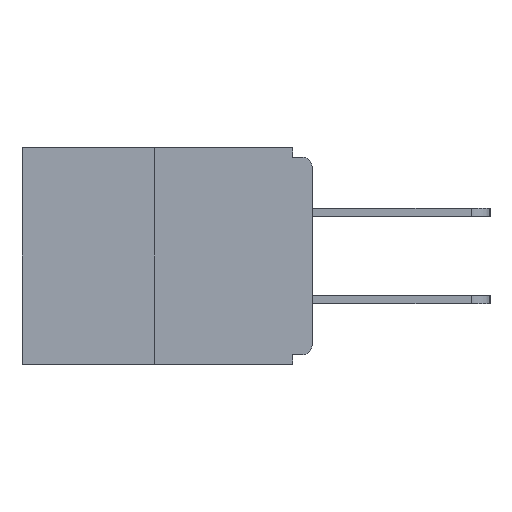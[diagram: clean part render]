
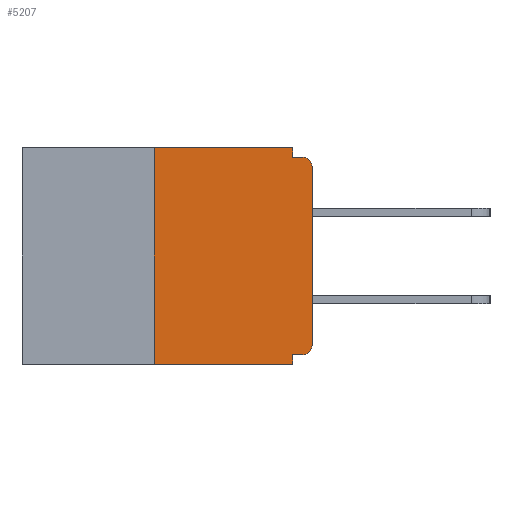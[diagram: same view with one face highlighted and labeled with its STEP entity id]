
A CAD part, left-side view. The second image highlights one B-rep face of the part: STEP entity #5207.
In plain terms, the highlighted planar face has unit normal (-1, 0, 0).
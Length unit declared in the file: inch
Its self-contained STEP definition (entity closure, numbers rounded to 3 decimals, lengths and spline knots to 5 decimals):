
#36 = ORIENTED_EDGE ( 'NONE', *, *, #3041, .F. ) ;
#191 = CARTESIAN_POINT ( 'NONE',  ( 0., 0.031, -0.328 ) ) ;
#299 = VECTOR ( 'NONE', #6464, 39.37008 ) ;
#502 = ORIENTED_EDGE ( 'NONE', *, *, #2843, .F. ) ;
#739 = EDGE_CURVE ( 'NONE', #14884, #6407, #12703, .T. ) ;
#771 = LINE ( 'NONE', #4756, #9662 ) ;
#773 = ORIENTED_EDGE ( 'NONE', *, *, #2170, .T. ) ;
#881 = LINE ( 'NONE', #10303, #8761 ) ;
#900 = LINE ( 'NONE', #12059, #10570 ) ;
#1342 = DIRECTION ( 'NONE',  ( 0., -1., 0. ) ) ;
#1424 = VERTEX_POINT ( 'NONE', #4488 ) ;
#1506 = VERTEX_POINT ( 'NONE', #13673 ) ;
#1543 = VERTEX_POINT ( 'NONE', #11147 ) ;
#1838 = ORIENTED_EDGE ( 'NONE', *, *, #739, .F. ) ;
#2103 = LINE ( 'NONE', #9027, #299 ) ;
#2170 = EDGE_CURVE ( 'NONE', #1424, #14766, #14477, .T. ) ;
#2428 = CARTESIAN_POINT ( 'NONE',  ( 0., 0.46, 0. ) ) ;
#2593 = VERTEX_POINT ( 'NONE', #6147 ) ;
#2674 = DIRECTION ( 'NONE',  ( 0., 0., -1. ) ) ;
#2838 = DIRECTION ( 'NONE',  ( 1., 0., 0. ) ) ;
#2843 = EDGE_CURVE ( 'NONE', #3686, #11981, #771, .T. ) ;
#3041 = EDGE_CURVE ( 'NONE', #1506, #1543, #13881, .T. ) ;
#3211 = CIRCLE ( 'NONE', #10064, 0.015 ) ;
#3686 = VERTEX_POINT ( 'NONE', #5465 ) ;
#3852 = DIRECTION ( 'NONE',  ( 0., 0., -1. ) ) ;
#4076 = AXIS2_PLACEMENT_3D ( 'NONE', #13822, #7461, #6131 ) ;
#4168 = DIRECTION ( 'NONE',  ( 0., 0., 1. ) ) ;
#4237 = EDGE_CURVE ( 'NONE', #14766, #2593, #5816, .T. ) ;
#4433 = ORIENTED_EDGE ( 'NONE', *, *, #15811, .T. ) ;
#4488 = CARTESIAN_POINT ( 'NONE',  ( 0., 0.015, -0.328 ) ) ;
#4657 = CARTESIAN_POINT ( 'NONE',  ( 0., 0.031, -0.343 ) ) ;
#4726 = EDGE_LOOP ( 'NONE', ( #36, #8362, #4433, #1838, #10491, #773, #16301, #13894, #502, #7622 ) ) ;
#4756 = CARTESIAN_POINT ( 'NONE',  ( 0., 0., -0.015 ) ) ;
#5207 = ADVANCED_FACE ( 'NONE', ( #11410 ), #7359, .F. ) ;
#5428 = DIRECTION ( 'NONE',  ( 0., 0., 1. ) ) ;
#5465 = CARTESIAN_POINT ( 'NONE',  ( 0., 0.031, -0.015 ) ) ;
#5483 = CARTESIAN_POINT ( 'NONE',  ( 0., 0., 0. ) ) ;
#5816 = LINE ( 'NONE', #5483, #12445 ) ;
#5883 = VECTOR ( 'NONE', #15792, 39.37008 ) ;
#6131 = DIRECTION ( 'NONE',  ( 0., 0., -1. ) ) ;
#6147 = CARTESIAN_POINT ( 'NONE',  ( 0., 0., -0.03 ) ) ;
#6407 = VERTEX_POINT ( 'NONE', #4657 ) ;
#6464 = DIRECTION ( 'NONE',  ( 0., 1., 0. ) ) ;
#6584 = CARTESIAN_POINT ( 'NONE',  ( 0., 0.015, -0.03 ) ) ;
#7234 = DIRECTION ( 'NONE',  ( 0., -1., 0. ) ) ;
#7359 = PLANE ( 'NONE',  #8649 ) ;
#7461 = DIRECTION ( 'NONE',  ( -1., 0., 0. ) ) ;
#7622 = ORIENTED_EDGE ( 'NONE', *, *, #11859, .F. ) ;
#8265 = VERTEX_POINT ( 'NONE', #16088 ) ;
#8362 = ORIENTED_EDGE ( 'NONE', *, *, #15459, .F. ) ;
#8649 = AXIS2_PLACEMENT_3D ( 'NONE', #10395, #2838, #2674 ) ;
#8681 = LINE ( 'NONE', #12797, #10885 ) ;
#8761 = VECTOR ( 'NONE', #1342, 39.37008 ) ;
#9027 = CARTESIAN_POINT ( 'NONE',  ( 0., 0., -0.328 ) ) ;
#9662 = VECTOR ( 'NONE', #7234, 39.37008 ) ;
#10064 = AXIS2_PLACEMENT_3D ( 'NONE', #6584, #12910, #15577 ) ;
#10303 = CARTESIAN_POINT ( 'NONE',  ( 0., 0.46, -0.343 ) ) ;
#10395 = CARTESIAN_POINT ( 'NONE',  ( 0., 0.46, 0. ) ) ;
#10491 = ORIENTED_EDGE ( 'NONE', *, *, #14849, .F. ) ;
#10570 = VECTOR ( 'NONE', #4168, 39.37008 ) ;
#10600 = CARTESIAN_POINT ( 'NONE',  ( 0., 0.031, -0.343 ) ) ;
#10885 = VECTOR ( 'NONE', #3852, 39.37008 ) ;
#11147 = CARTESIAN_POINT ( 'NONE',  ( 0., 0.031, 0. ) ) ;
#11410 = FACE_OUTER_BOUND ( 'NONE', #4726, .T. ) ;
#11806 = EDGE_CURVE ( 'NONE', #2593, #11981, #3211, .T. ) ;
#11859 = EDGE_CURVE ( 'NONE', #1543, #3686, #8681, .T. ) ;
#11981 = VERTEX_POINT ( 'NONE', #13239 ) ;
#12059 = CARTESIAN_POINT ( 'NONE',  ( 0., 0.25, 0. ) ) ;
#12445 = VECTOR ( 'NONE', #5428, 39.37008 ) ;
#12703 = LINE ( 'NONE', #10600, #5883 ) ;
#12797 = CARTESIAN_POINT ( 'NONE',  ( 0., 0.031, 0. ) ) ;
#12910 = DIRECTION ( 'NONE',  ( -1., 0., 0. ) ) ;
#13239 = CARTESIAN_POINT ( 'NONE',  ( 0., 0.015, -0.015 ) ) ;
#13673 = CARTESIAN_POINT ( 'NONE',  ( 0., 0.25, 0. ) ) ;
#13822 = CARTESIAN_POINT ( 'NONE',  ( 0., 0.015, -0.313 ) ) ;
#13881 = LINE ( 'NONE', #2428, #14878 ) ;
#13894 = ORIENTED_EDGE ( 'NONE', *, *, #11806, .T. ) ;
#13994 = CARTESIAN_POINT ( 'NONE',  ( 0., 0., -0.313 ) ) ;
#14477 = CIRCLE ( 'NONE', #4076, 0.015 ) ;
#14766 = VERTEX_POINT ( 'NONE', #13994 ) ;
#14849 = EDGE_CURVE ( 'NONE', #1424, #14884, #2103, .T. ) ;
#14878 = VECTOR ( 'NONE', #15226, 39.37008 ) ;
#14884 = VERTEX_POINT ( 'NONE', #191 ) ;
#15226 = DIRECTION ( 'NONE',  ( 0., -1., 0. ) ) ;
#15459 = EDGE_CURVE ( 'NONE', #8265, #1506, #900, .T. ) ;
#15577 = DIRECTION ( 'NONE',  ( 0., 0., -1. ) ) ;
#15792 = DIRECTION ( 'NONE',  ( 0., 0., -1. ) ) ;
#15811 = EDGE_CURVE ( 'NONE', #8265, #6407, #881, .T. ) ;
#16088 = CARTESIAN_POINT ( 'NONE',  ( 0., 0.25, -0.343 ) ) ;
#16301 = ORIENTED_EDGE ( 'NONE', *, *, #4237, .T. ) ;
